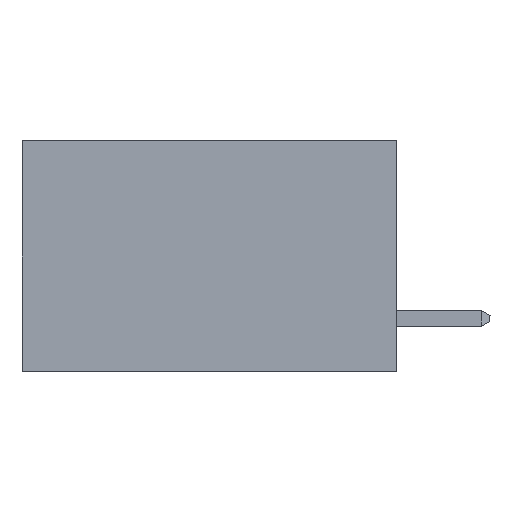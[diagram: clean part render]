
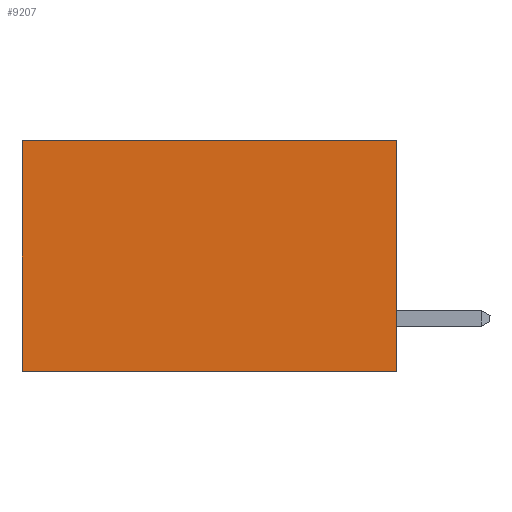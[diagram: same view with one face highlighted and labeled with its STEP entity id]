
A CAD part, left-side view. The second image highlights one B-rep face of the part: STEP entity #9207.
In plain terms, the highlighted planar face has unit normal (-1, 0, 0).
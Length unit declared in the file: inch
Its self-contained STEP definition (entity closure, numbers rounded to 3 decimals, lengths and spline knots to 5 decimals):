
#58 = CARTESIAN_POINT ( 'NONE',  ( 0.2615, 0., 0. ) ) ;
#141 = LINE ( 'NONE', #10971, #4664 ) ;
#230 = VECTOR ( 'NONE', #8453, 39.37008 ) ;
#378 = CARTESIAN_POINT ( 'NONE',  ( 0.2615, 0.6, 0. ) ) ;
#727 = CARTESIAN_POINT ( 'NONE',  ( 0.2615, 0., -0.37 ) ) ;
#1410 = LINE ( 'NONE', #9442, #230 ) ;
#3311 = DIRECTION ( 'NONE',  ( 0., 0., -1. ) ) ;
#3804 = DIRECTION ( 'NONE',  ( 1., 0., 0. ) ) ;
#3890 = ORIENTED_EDGE ( 'NONE', *, *, #8091, .T. ) ;
#4015 = ORIENTED_EDGE ( 'NONE', *, *, #9897, .F. ) ;
#4441 = EDGE_CURVE ( 'NONE', #5583, #9845, #141, .T. ) ;
#4664 = VECTOR ( 'NONE', #7137, 39.37008 ) ;
#4952 = DIRECTION ( 'NONE',  ( 0., 0., -1. ) ) ;
#5141 = VERTEX_POINT ( 'NONE', #8476 ) ;
#5331 = CARTESIAN_POINT ( 'NONE',  ( 0.2615, 0., -0.37 ) ) ;
#5393 = LINE ( 'NONE', #5331, #9595 ) ;
#5583 = VERTEX_POINT ( 'NONE', #8780 ) ;
#5638 = AXIS2_PLACEMENT_3D ( 'NONE', #727, #3804, #4952 ) ;
#5812 = FACE_OUTER_BOUND ( 'NONE', #6972, .T. ) ;
#6040 = CARTESIAN_POINT ( 'NONE',  ( 0.2615, 0.6, -0.37 ) ) ;
#6846 = VERTEX_POINT ( 'NONE', #378 ) ;
#6860 = PLANE ( 'NONE',  #5638 ) ;
#6972 = EDGE_LOOP ( 'NONE', ( #12714, #8876, #4015, #3890 ) ) ;
#7040 = LINE ( 'NONE', #58, #9133 ) ;
#7137 = DIRECTION ( 'NONE',  ( 0., 1., 0. ) ) ;
#8091 = EDGE_CURVE ( 'NONE', #5141, #6846, #7040, .T. ) ;
#8453 = DIRECTION ( 'NONE',  ( 0., 0., -1. ) ) ;
#8476 = CARTESIAN_POINT ( 'NONE',  ( 0.2615, 0., 0. ) ) ;
#8780 = CARTESIAN_POINT ( 'NONE',  ( 0.2615, 0., -0.37 ) ) ;
#8876 = ORIENTED_EDGE ( 'NONE', *, *, #4441, .F. ) ;
#9133 = VECTOR ( 'NONE', #12193, 39.37008 ) ;
#9207 = ADVANCED_FACE ( 'NONE', ( #5812 ), #6860, .F. ) ;
#9442 = CARTESIAN_POINT ( 'NONE',  ( 0.2615, 0.6, -0.37 ) ) ;
#9595 = VECTOR ( 'NONE', #3311, 39.37008 ) ;
#9845 = VERTEX_POINT ( 'NONE', #6040 ) ;
#9897 = EDGE_CURVE ( 'NONE', #5141, #5583, #5393, .T. ) ;
#10971 = CARTESIAN_POINT ( 'NONE',  ( 0.2615, 0., -0.37 ) ) ;
#12193 = DIRECTION ( 'NONE',  ( 0., 1., 0. ) ) ;
#12457 = EDGE_CURVE ( 'NONE', #6846, #9845, #1410, .T. ) ;
#12714 = ORIENTED_EDGE ( 'NONE', *, *, #12457, .T. ) ;
